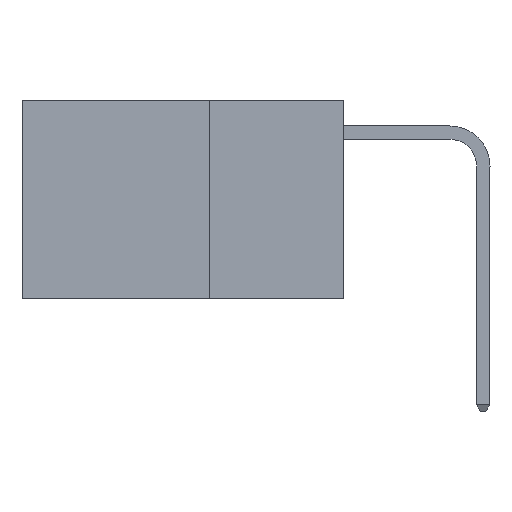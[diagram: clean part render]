
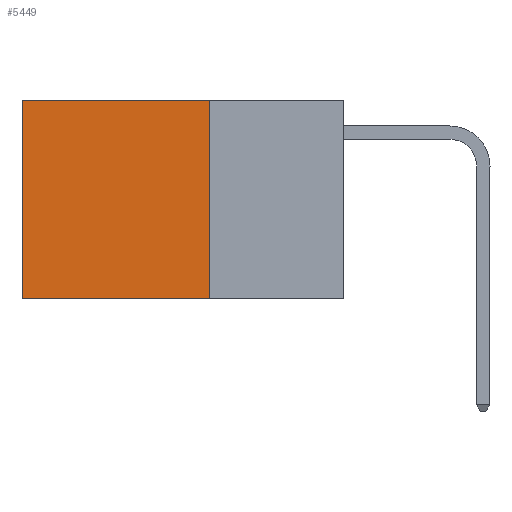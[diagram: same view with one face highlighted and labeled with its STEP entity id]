
A CAD part, left-side view. The second image highlights one B-rep face of the part: STEP entity #5449.
In plain terms, the highlighted planar face has unit normal (-1, 0, 0).
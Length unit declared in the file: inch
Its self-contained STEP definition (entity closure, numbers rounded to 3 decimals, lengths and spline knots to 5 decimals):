
#961 = CARTESIAN_POINT ( 'NONE',  ( 0.2625, 0.25, 0. ) ) ;
#1028 = EDGE_CURVE ( 'NONE', #8310, #9515, #8736, .T. ) ;
#1323 = CARTESIAN_POINT ( 'NONE',  ( 0.2625, 0.25, 0. ) ) ;
#1407 = LINE ( 'NONE', #9128, #6790 ) ;
#2140 = VERTEX_POINT ( 'NONE', #6449 ) ;
#2471 = DIRECTION ( 'NONE',  ( 1., 0., 0. ) ) ;
#2766 = CARTESIAN_POINT ( 'NONE',  ( 0.2625, 0.25, 0. ) ) ;
#3088 = EDGE_CURVE ( 'NONE', #8310, #10969, #9835, .T. ) ;
#4375 = ORIENTED_EDGE ( 'NONE', *, *, #5831, .F. ) ;
#4649 = ORIENTED_EDGE ( 'NONE', *, *, #12392, .T. ) ;
#4667 = ORIENTED_EDGE ( 'NONE', *, *, #3088, .T. ) ;
#4991 = ORIENTED_EDGE ( 'NONE', *, *, #1028, .F. ) ;
#5117 = CARTESIAN_POINT ( 'NONE',  ( 0.2625, 0.25, -0.37 ) ) ;
#5449 = ADVANCED_FACE ( 'NONE', ( #8966 ), #8711, .F. ) ;
#5544 = DIRECTION ( 'NONE',  ( 0., 0., -1. ) ) ;
#5618 = AXIS2_PLACEMENT_3D ( 'NONE', #1323, #2471, #9748 ) ;
#5831 = EDGE_CURVE ( 'NONE', #9515, #2140, #13090, .T. ) ;
#6069 = VECTOR ( 'NONE', #5544, 39.37008 ) ;
#6449 = CARTESIAN_POINT ( 'NONE',  ( 0.2625, 0.6, -0.37 ) ) ;
#6621 = CARTESIAN_POINT ( 'NONE',  ( 0.2625, 0.6, 0. ) ) ;
#6790 = VECTOR ( 'NONE', #10186, 39.37008 ) ;
#7425 = VECTOR ( 'NONE', #9973, 39.37008 ) ;
#7701 = VECTOR ( 'NONE', #13296, 39.37008 ) ;
#8310 = VERTEX_POINT ( 'NONE', #961 ) ;
#8711 = PLANE ( 'NONE',  #5618 ) ;
#8736 = LINE ( 'NONE', #8757, #6069 ) ;
#8755 = EDGE_LOOP ( 'NONE', ( #4649, #4375, #4991, #4667 ) ) ;
#8757 = CARTESIAN_POINT ( 'NONE',  ( 0.2625, 0.25, 0. ) ) ;
#8966 = FACE_OUTER_BOUND ( 'NONE', #8755, .T. ) ;
#9128 = CARTESIAN_POINT ( 'NONE',  ( 0.2625, 0.6, 0. ) ) ;
#9515 = VERTEX_POINT ( 'NONE', #5117 ) ;
#9748 = DIRECTION ( 'NONE',  ( 0., 0., -1. ) ) ;
#9835 = LINE ( 'NONE', #2766, #7425 ) ;
#9973 = DIRECTION ( 'NONE',  ( 0., 1., 0. ) ) ;
#10186 = DIRECTION ( 'NONE',  ( 0., 0., -1. ) ) ;
#10969 = VERTEX_POINT ( 'NONE', #6621 ) ;
#11371 = CARTESIAN_POINT ( 'NONE',  ( 0.2625, 0.25, -0.37 ) ) ;
#12392 = EDGE_CURVE ( 'NONE', #10969, #2140, #1407, .T. ) ;
#13090 = LINE ( 'NONE', #11371, #7701 ) ;
#13296 = DIRECTION ( 'NONE',  ( 0., 1., 0. ) ) ;
